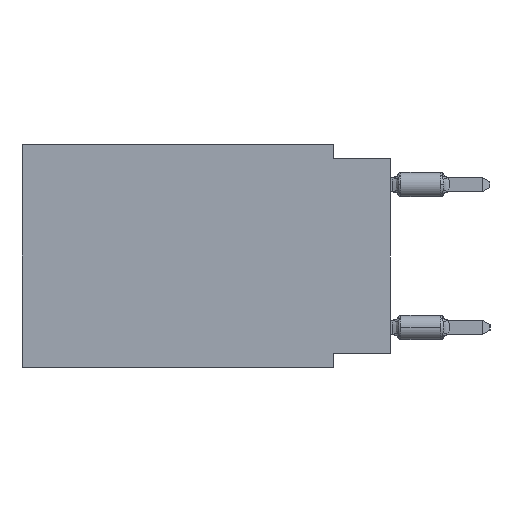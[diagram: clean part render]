
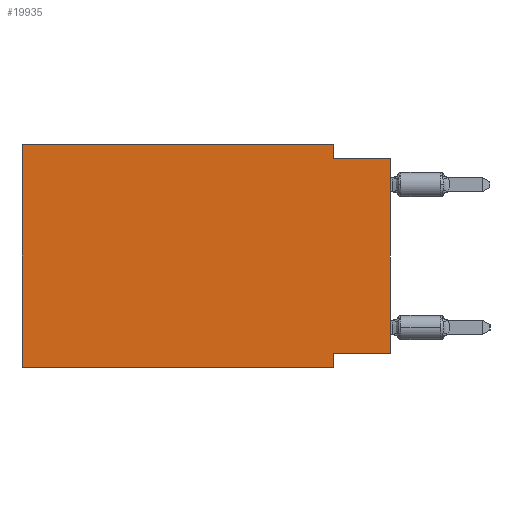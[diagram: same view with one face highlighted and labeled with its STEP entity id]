
A CAD part, left-side view. The second image highlights one B-rep face of the part: STEP entity #19935.
In plain terms, the highlighted planar face has unit normal (-1, 0, 0).
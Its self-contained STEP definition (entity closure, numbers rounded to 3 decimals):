
#609 = VERTEX_POINT ( 'NONE', #2331 ) ;
#720 = ORIENTED_EDGE ( 'NONE', *, *, #26189, .F. ) ;
#2331 = CARTESIAN_POINT ( 'NONE',  ( 0., 2.54, -0.635 ) ) ;
#3654 = CARTESIAN_POINT ( 'NONE',  ( 0., 2.54, -9.906 ) ) ;
#4836 = EDGE_CURVE ( 'NONE', #609, #42502, #9949, .T. ) ;
#5219 = DIRECTION ( 'NONE',  ( 0., 1., 0. ) ) ;
#5760 = EDGE_CURVE ( 'NONE', #24839, #31168, #10500, .T. ) ;
#6326 = VERTEX_POINT ( 'NONE', #32587 ) ;
#6729 = DIRECTION ( 'NONE',  ( 0., -1., 0. ) ) ;
#7807 = ORIENTED_EDGE ( 'NONE', *, *, #17498, .F. ) ;
#8041 = LINE ( 'NONE', #38923, #28022 ) ;
#8558 = LINE ( 'NONE', #22055, #20593 ) ;
#9293 = ORIENTED_EDGE ( 'NONE', *, *, #5760, .F. ) ;
#9949 = LINE ( 'NONE', #27777, #36867 ) ;
#10500 = LINE ( 'NONE', #10945, #26733 ) ;
#10832 = CARTESIAN_POINT ( 'NONE',  ( 0., 2.54, 0. ) ) ;
#10938 = DIRECTION ( 'NONE',  ( 0., 0., -1. ) ) ;
#10945 = CARTESIAN_POINT ( 'NONE',  ( 0., 2.54, -9.906 ) ) ;
#11242 = VECTOR ( 'NONE', #5219, 1000. ) ;
#11256 = EDGE_LOOP ( 'NONE', ( #13859, #33590, #29364, #7807, #720, #16076, #9293, #18315 ) ) ;
#11340 = VECTOR ( 'NONE', #36134, 1000. ) ;
#12994 = CARTESIAN_POINT ( 'NONE',  ( 0., 2.54, -9.271 ) ) ;
#13859 = ORIENTED_EDGE ( 'NONE', *, *, #40776, .T. ) ;
#15774 = DIRECTION ( 'NONE',  ( 0., 0., 1. ) ) ;
#16076 = ORIENTED_EDGE ( 'NONE', *, *, #24940, .T. ) ;
#17498 = EDGE_CURVE ( 'NONE', #6326, #19006, #42652, .T. ) ;
#17658 = CARTESIAN_POINT ( 'NONE',  ( 0., 0., -9.271 ) ) ;
#17817 = PLANE ( 'NONE',  #27326 ) ;
#18102 = LINE ( 'NONE', #35891, #11340 ) ;
#18315 = ORIENTED_EDGE ( 'NONE', *, *, #32669, .F. ) ;
#18471 = FACE_OUTER_BOUND ( 'NONE', #11256, .T. ) ;
#19006 = VERTEX_POINT ( 'NONE', #10832 ) ;
#19935 = ADVANCED_FACE ( 'NONE', ( #18471 ), #17817, .F. ) ;
#20593 = VECTOR ( 'NONE', #33003, 1000. ) ;
#20772 = EDGE_CURVE ( 'NONE', #19006, #609, #18102, .T. ) ;
#20914 = CARTESIAN_POINT ( 'NONE',  ( 0., 16.383, -9.906 ) ) ;
#21327 = DIRECTION ( 'NONE',  ( 0., 0., 1. ) ) ;
#21537 = VECTOR ( 'NONE', #15774, 1000. ) ;
#22055 = CARTESIAN_POINT ( 'NONE',  ( 0., 16.383, -9.906 ) ) ;
#22630 = VERTEX_POINT ( 'NONE', #20914 ) ;
#23075 = CARTESIAN_POINT ( 'NONE',  ( 0., 0., 0. ) ) ;
#23283 = LINE ( 'NONE', #23075, #21537 ) ;
#24839 = VERTEX_POINT ( 'NONE', #12994 ) ;
#24940 = EDGE_CURVE ( 'NONE', #22630, #31168, #8558, .T. ) ;
#25117 = CARTESIAN_POINT ( 'NONE',  ( 0., 16.383, 0. ) ) ;
#26189 = EDGE_CURVE ( 'NONE', #22630, #6326, #8041, .T. ) ;
#26733 = VECTOR ( 'NONE', #38819, 1000. ) ;
#27326 = AXIS2_PLACEMENT_3D ( 'NONE', #25117, #35626, #10938 ) ;
#27777 = CARTESIAN_POINT ( 'NONE',  ( 0., 0., -0.635 ) ) ;
#28022 = VECTOR ( 'NONE', #21327, 1000. ) ;
#29364 = ORIENTED_EDGE ( 'NONE', *, *, #20772, .F. ) ;
#30393 = LINE ( 'NONE', #36547, #11242 ) ;
#31168 = VERTEX_POINT ( 'NONE', #3654 ) ;
#32114 = CARTESIAN_POINT ( 'NONE',  ( 0., 16.383, 0. ) ) ;
#32195 = VECTOR ( 'NONE', #39636, 1000. ) ;
#32587 = CARTESIAN_POINT ( 'NONE',  ( 0., 16.383, 0. ) ) ;
#32669 = EDGE_CURVE ( 'NONE', #41155, #24839, #30393, .T. ) ;
#33003 = DIRECTION ( 'NONE',  ( 0., -1., 0. ) ) ;
#33590 = ORIENTED_EDGE ( 'NONE', *, *, #4836, .F. ) ;
#35626 = DIRECTION ( 'NONE',  ( 1., 0., 0. ) ) ;
#35891 = CARTESIAN_POINT ( 'NONE',  ( 0., 2.54, 0. ) ) ;
#36134 = DIRECTION ( 'NONE',  ( 0., 0., -1. ) ) ;
#36547 = CARTESIAN_POINT ( 'NONE',  ( 0., 0., -9.271 ) ) ;
#36867 = VECTOR ( 'NONE', #6729, 1000. ) ;
#38819 = DIRECTION ( 'NONE',  ( 0., 0., -1. ) ) ;
#38923 = CARTESIAN_POINT ( 'NONE',  ( 0., 16.383, 0. ) ) ;
#39636 = DIRECTION ( 'NONE',  ( 0., -1., 0. ) ) ;
#40715 = CARTESIAN_POINT ( 'NONE',  ( 0., 0., -0.635 ) ) ;
#40776 = EDGE_CURVE ( 'NONE', #41155, #42502, #23283, .T. ) ;
#41155 = VERTEX_POINT ( 'NONE', #17658 ) ;
#42502 = VERTEX_POINT ( 'NONE', #40715 ) ;
#42652 = LINE ( 'NONE', #32114, #32195 ) ;
